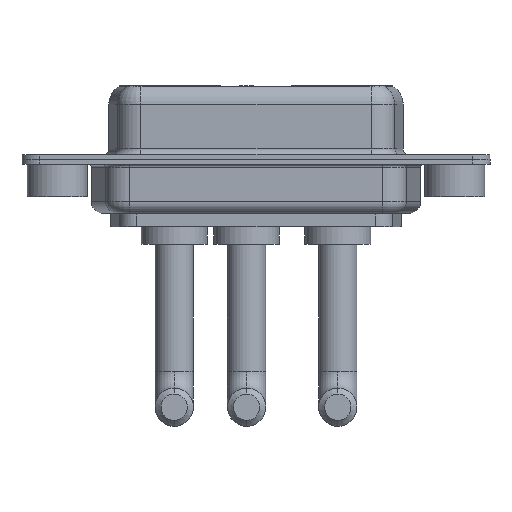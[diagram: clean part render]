
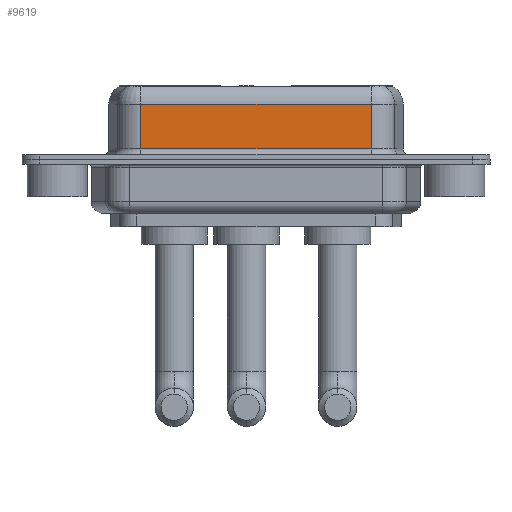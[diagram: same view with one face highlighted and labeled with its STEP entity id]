
A CAD part, front view. The second image highlights one B-rep face of the part: STEP entity #9619.
In plain terms, the highlighted planar face has unit normal (0, -1, 0).
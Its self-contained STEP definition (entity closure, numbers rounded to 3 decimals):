
#78 = DIRECTION ( 'NONE',  ( 1., 0., 0. ) ) ;
#95 = VECTOR ( 'NONE', #8559, 1000. ) ;
#340 = AXIS2_PLACEMENT_3D ( 'NONE', #6199, #11424, #8222 ) ;
#481 = DIRECTION ( 'NONE',  ( 0., 0., -1. ) ) ;
#1016 = EDGE_CURVE ( 'NONE', #7942, #5762, #12820, .T. ) ;
#1675 = DIRECTION ( 'NONE',  ( -1., 0., 0. ) ) ;
#2178 = VERTEX_POINT ( 'NONE', #10951 ) ;
#2243 = CARTESIAN_POINT ( 'NONE',  ( 26.287, -3.95, 0.9 ) ) ;
#2517 = CARTESIAN_POINT ( 'NONE',  ( 26.287, -3.95, 4.65 ) ) ;
#2780 = LINE ( 'NONE', #7020, #3931 ) ;
#2954 = VERTEX_POINT ( 'NONE', #5819 ) ;
#3760 = ORIENTED_EDGE ( 'NONE', *, *, #12950, .F. ) ;
#3931 = VECTOR ( 'NONE', #481, 1000. ) ;
#3934 = VECTOR ( 'NONE', #1675, 1000. ) ;
#4440 = CARTESIAN_POINT ( 'NONE',  ( 26.287, -3.95, 0.9 ) ) ;
#5343 = CARTESIAN_POINT ( 'NONE',  ( 7.013, -3.95, 0.9 ) ) ;
#5762 = VERTEX_POINT ( 'NONE', #2243 ) ;
#5819 = CARTESIAN_POINT ( 'NONE',  ( 26.287, -3.95, 4.65 ) ) ;
#6199 = CARTESIAN_POINT ( 'NONE',  ( 26.287, -3.95, 6.4 ) ) ;
#6280 = VECTOR ( 'NONE', #78, 1000. ) ;
#6396 = CARTESIAN_POINT ( 'NONE',  ( 7.013, -3.95, 6.4 ) ) ;
#6568 = ORIENTED_EDGE ( 'NONE', *, *, #11346, .T. ) ;
#7020 = CARTESIAN_POINT ( 'NONE',  ( 26.287, -3.95, 6.4 ) ) ;
#7124 = EDGE_LOOP ( 'NONE', ( #3760, #6568, #9346, #10668 ) ) ;
#7179 = FACE_OUTER_BOUND ( 'NONE', #7124, .T. ) ;
#7942 = VERTEX_POINT ( 'NONE', #5343 ) ;
#8222 = DIRECTION ( 'NONE',  ( 0., 0., 1. ) ) ;
#8492 = LINE ( 'NONE', #6396, #95 ) ;
#8559 = DIRECTION ( 'NONE',  ( 0., 0., -1. ) ) ;
#9061 = LINE ( 'NONE', #2517, #3934 ) ;
#9129 = EDGE_CURVE ( 'NONE', #2178, #7942, #8492, .T. ) ;
#9346 = ORIENTED_EDGE ( 'NONE', *, *, #9129, .T. ) ;
#9619 = ADVANCED_FACE ( 'NONE', ( #7179 ), #13519, .F. ) ;
#10668 = ORIENTED_EDGE ( 'NONE', *, *, #1016, .T. ) ;
#10951 = CARTESIAN_POINT ( 'NONE',  ( 7.013, -3.95, 4.65 ) ) ;
#11346 = EDGE_CURVE ( 'NONE', #2954, #2178, #9061, .T. ) ;
#11424 = DIRECTION ( 'NONE',  ( 0., 1., 0. ) ) ;
#12820 = LINE ( 'NONE', #4440, #6280 ) ;
#12950 = EDGE_CURVE ( 'NONE', #2954, #5762, #2780, .T. ) ;
#13519 = PLANE ( 'NONE',  #340 ) ;
